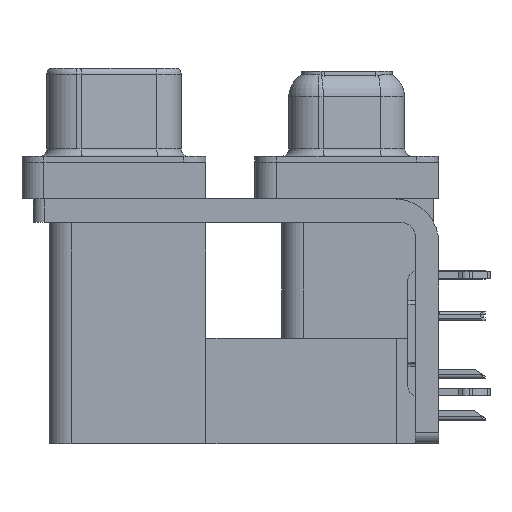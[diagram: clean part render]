
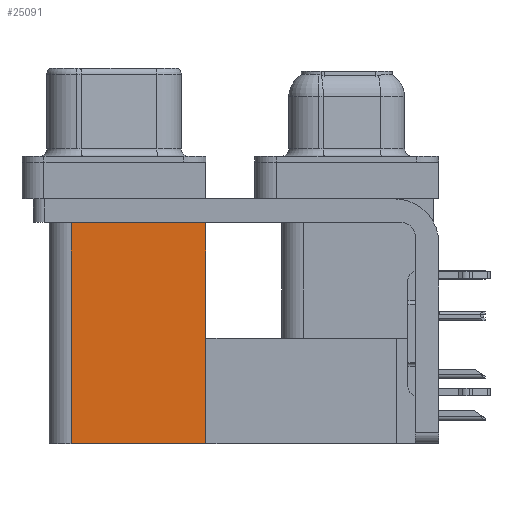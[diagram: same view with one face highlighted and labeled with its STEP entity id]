
A CAD part, left-side view. The second image highlights one B-rep face of the part: STEP entity #25091.
In plain terms, the highlighted planar face has unit normal (-1, 0, 0).
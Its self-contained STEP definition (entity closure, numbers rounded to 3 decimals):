
#953 = VECTOR ( 'NONE', #44087, 1000. ) ;
#3141 = CARTESIAN_POINT ( 'NONE',  ( 3.765, 9.6, -19.2 ) ) ;
#3579 = EDGE_LOOP ( 'NONE', ( #42893, #6603, #20416, #25170 ) ) ;
#3585 = CARTESIAN_POINT ( 'NONE',  ( 3.765, 9.6, -2.5 ) ) ;
#6603 = ORIENTED_EDGE ( 'NONE', *, *, #19294, .F. ) ;
#8564 = CARTESIAN_POINT ( 'NONE',  ( 3.765, 18.8, -19.2 ) ) ;
#10549 = DIRECTION ( 'NONE',  ( 0., 1., 0. ) ) ;
#13378 = FACE_OUTER_BOUND ( 'NONE', #3579, .T. ) ;
#14095 = CARTESIAN_POINT ( 'NONE',  ( 3.765, 18.8, -19.2 ) ) ;
#14489 = CARTESIAN_POINT ( 'NONE',  ( 3.765, 9.6, -19.2 ) ) ;
#14748 = VECTOR ( 'NONE', #10549, 1000. ) ;
#16944 = PLANE ( 'NONE',  #43025 ) ;
#19267 = CARTESIAN_POINT ( 'NONE',  ( 3.765, 18.8, -2.5 ) ) ;
#19294 = EDGE_CURVE ( 'NONE', #39606, #24738, #41790, .T. ) ;
#19393 = CARTESIAN_POINT ( 'NONE',  ( 3.765, 9.6, -19.2 ) ) ;
#20416 = ORIENTED_EDGE ( 'NONE', *, *, #20901, .F. ) ;
#20901 = EDGE_CURVE ( 'NONE', #28785, #39606, #27480, .T. ) ;
#24738 = VERTEX_POINT ( 'NONE', #19267 ) ;
#24747 = CARTESIAN_POINT ( 'NONE',  ( 3.765, 9.6, -2.5 ) ) ;
#25091 = ADVANCED_FACE ( 'NONE', ( #13378 ), #16944, .F. ) ;
#25170 = ORIENTED_EDGE ( 'NONE', *, *, #26489, .T. ) ;
#25753 = LINE ( 'NONE', #3141, #953 ) ;
#26489 = EDGE_CURVE ( 'NONE', #28785, #28394, #25753, .T. ) ;
#26697 = CARTESIAN_POINT ( 'NONE',  ( 3.765, 9.6, -19.2 ) ) ;
#26773 = VECTOR ( 'NONE', #41751, 1000. ) ;
#27480 = LINE ( 'NONE', #14489, #26773 ) ;
#28394 = VERTEX_POINT ( 'NONE', #24747 ) ;
#28785 = VERTEX_POINT ( 'NONE', #26697 ) ;
#33706 = DIRECTION ( 'NONE',  ( 0., 0., -1. ) ) ;
#36880 = LINE ( 'NONE', #3585, #14748 ) ;
#39606 = VERTEX_POINT ( 'NONE', #8564 ) ;
#39963 = DIRECTION ( 'NONE',  ( 1., 0., 0. ) ) ;
#41348 = DIRECTION ( 'NONE',  ( 0., 0., 1. ) ) ;
#41637 = VECTOR ( 'NONE', #41348, 1000. ) ;
#41751 = DIRECTION ( 'NONE',  ( 0., 1., 0. ) ) ;
#41790 = LINE ( 'NONE', #14095, #41637 ) ;
#42117 = EDGE_CURVE ( 'NONE', #28394, #24738, #36880, .T. ) ;
#42893 = ORIENTED_EDGE ( 'NONE', *, *, #42117, .T. ) ;
#43025 = AXIS2_PLACEMENT_3D ( 'NONE', #19393, #39963, #33706 ) ;
#44087 = DIRECTION ( 'NONE',  ( 0., 0., 1. ) ) ;
